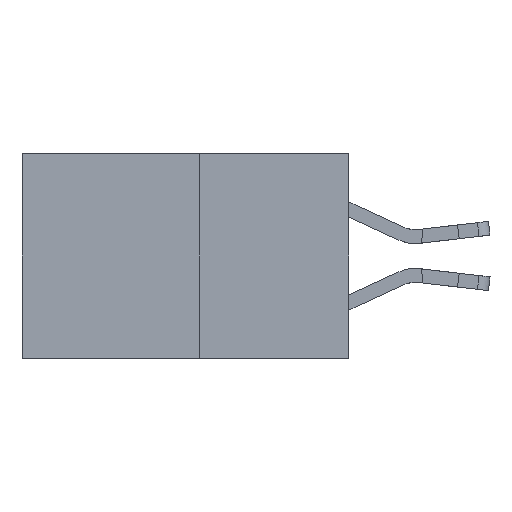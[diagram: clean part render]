
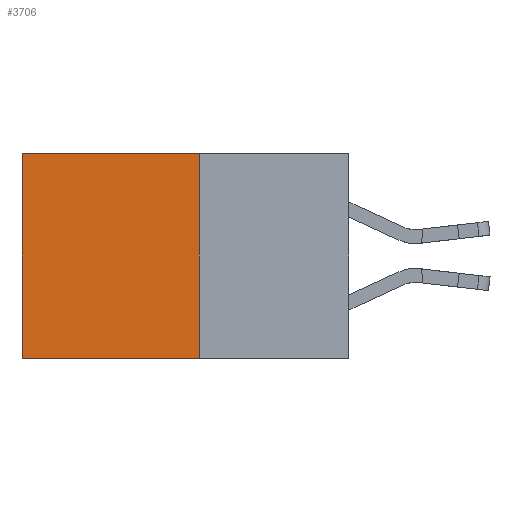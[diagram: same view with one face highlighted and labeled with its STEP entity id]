
A CAD part, left-side view. The second image highlights one B-rep face of the part: STEP entity #3706.
In plain terms, the highlighted planar face has unit normal (-1, 0, 0).
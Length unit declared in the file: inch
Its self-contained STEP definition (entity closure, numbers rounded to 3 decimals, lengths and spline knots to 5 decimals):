
#249 = DIRECTION ( 'NONE',  ( 0., 0., -1. ) ) ;
#832 = ORIENTED_EDGE ( 'NONE', *, *, #15249, .T. ) ;
#1087 = VECTOR ( 'NONE', #249, 39.37008 ) ;
#1149 = VERTEX_POINT ( 'NONE', #10704 ) ;
#1472 = AXIS2_PLACEMENT_3D ( 'NONE', #4047, #4138, #4158 ) ;
#1621 = EDGE_CURVE ( 'NONE', #1149, #2940, #5862, .T. ) ;
#1673 = CARTESIAN_POINT ( 'NONE',  ( 0.277, 0.59, -0.37 ) ) ;
#2012 = ORIENTED_EDGE ( 'NONE', *, *, #1621, .F. ) ;
#2075 = FACE_OUTER_BOUND ( 'NONE', #11378, .T. ) ;
#2919 = CARTESIAN_POINT ( 'NONE',  ( 0.277, 0.59, 0. ) ) ;
#2940 = VERTEX_POINT ( 'NONE', #1673 ) ;
#3028 = DIRECTION ( 'NONE',  ( 0., 0., -1. ) ) ;
#3706 = ADVANCED_FACE ( 'NONE', ( #2075 ), #4051, .F. ) ;
#3714 = DIRECTION ( 'NONE',  ( 0., 1., 0. ) ) ;
#3732 = CARTESIAN_POINT ( 'NONE',  ( 0.277, 0.27, -0.37 ) ) ;
#4047 = CARTESIAN_POINT ( 'NONE',  ( 0.277, 0.27, -0.37 ) ) ;
#4051 = PLANE ( 'NONE',  #1472 ) ;
#4138 = DIRECTION ( 'NONE',  ( 1., 0., 0. ) ) ;
#4158 = DIRECTION ( 'NONE',  ( 0., 0., -1. ) ) ;
#4234 = ORIENTED_EDGE ( 'NONE', *, *, #8252, .T. ) ;
#4537 = CARTESIAN_POINT ( 'NONE',  ( 0.277, 0.27, 0. ) ) ;
#5862 = LINE ( 'NONE', #3732, #15234 ) ;
#6570 = VERTEX_POINT ( 'NONE', #2919 ) ;
#6866 = CARTESIAN_POINT ( 'NONE',  ( 0.277, 0.59, -0.37 ) ) ;
#7370 = VECTOR ( 'NONE', #3028, 39.37008 ) ;
#8252 = EDGE_CURVE ( 'NONE', #6570, #2940, #13880, .T. ) ;
#8319 = VERTEX_POINT ( 'NONE', #15004 ) ;
#8351 = DIRECTION ( 'NONE',  ( 0., 1., 0. ) ) ;
#9593 = ORIENTED_EDGE ( 'NONE', *, *, #13887, .F. ) ;
#10286 = LINE ( 'NONE', #13840, #1087 ) ;
#10704 = CARTESIAN_POINT ( 'NONE',  ( 0.277, 0.27, -0.37 ) ) ;
#11378 = EDGE_LOOP ( 'NONE', ( #4234, #2012, #9593, #832 ) ) ;
#13840 = CARTESIAN_POINT ( 'NONE',  ( 0.277, 0.27, -0.37 ) ) ;
#13880 = LINE ( 'NONE', #6866, #7370 ) ;
#13887 = EDGE_CURVE ( 'NONE', #8319, #1149, #10286, .T. ) ;
#14695 = VECTOR ( 'NONE', #8351, 39.37008 ) ;
#15004 = CARTESIAN_POINT ( 'NONE',  ( 0.277, 0.27, 0. ) ) ;
#15234 = VECTOR ( 'NONE', #3714, 39.37008 ) ;
#15249 = EDGE_CURVE ( 'NONE', #8319, #6570, #15431, .T. ) ;
#15431 = LINE ( 'NONE', #4537, #14695 ) ;
